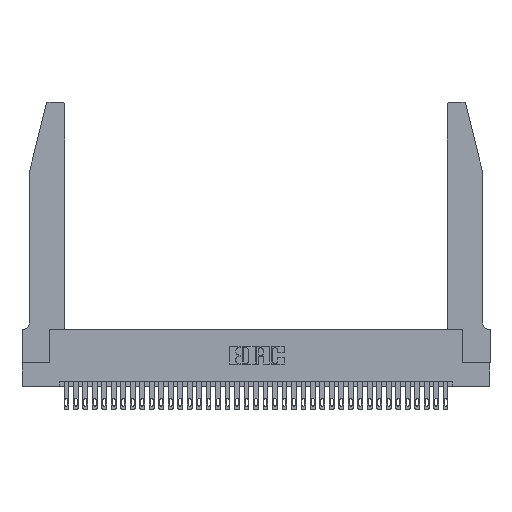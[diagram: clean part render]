
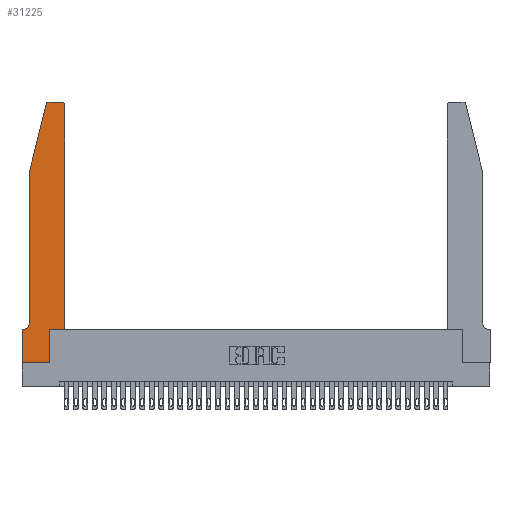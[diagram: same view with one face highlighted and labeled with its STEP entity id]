
A CAD part, top view. The second image highlights one B-rep face of the part: STEP entity #31225.
In plain terms, the highlighted planar face has unit normal (0, 0, 1).
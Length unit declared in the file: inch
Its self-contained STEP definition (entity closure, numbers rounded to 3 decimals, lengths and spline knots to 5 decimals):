
#162 = LINE ( 'NONE', #22549, #29637 ) ;
#183 = DIRECTION ( 'NONE',  ( 0., -1., 0. ) ) ;
#596 = CARTESIAN_POINT ( 'NONE',  ( 0.4205, 2.72, 0.37 ) ) ;
#1191 = VERTEX_POINT ( 'NONE', #33438 ) ;
#1701 = EDGE_CURVE ( 'NONE', #1191, #5198, #1761, .T. ) ;
#1761 = LINE ( 'NONE', #12296, #34817 ) ;
#2145 = VECTOR ( 'NONE', #18268, 39.37008 ) ;
#2172 = CIRCLE ( 'NONE', #9292, 0.03 ) ;
#2718 = VECTOR ( 'NONE', #27324, 39.37008 ) ;
#3950 = CARTESIAN_POINT ( 'NONE',  ( 0.2865, 0., 0.37 ) ) ;
#4523 = LINE ( 'NONE', #21981, #15677 ) ;
#5197 = DIRECTION ( 'NONE',  ( -0.239, -0.971, 0. ) ) ;
#5198 = VERTEX_POINT ( 'NONE', #32969 ) ;
#5276 = ORIENTED_EDGE ( 'NONE', *, *, #17188, .T. ) ;
#6531 = DIRECTION ( 'NONE',  ( 1., 0., 0. ) ) ;
#6892 = EDGE_CURVE ( 'NONE', #14827, #27369, #30427, .T. ) ;
#7015 = CARTESIAN_POINT ( 'NONE',  ( 0.0055, 0.42, 0.37 ) ) ;
#7888 = DIRECTION ( 'NONE',  ( 0., -1., 0. ) ) ;
#8024 = LINE ( 'NONE', #29529, #2145 ) ;
#8298 = CARTESIAN_POINT ( 'NONE',  ( 0.0755, 2., 0.37 ) ) ;
#9032 = ORIENTED_EDGE ( 'NONE', *, *, #20351, .T. ) ;
#9292 = AXIS2_PLACEMENT_3D ( 'NONE', #596, #12249, #28972 ) ;
#9358 = AXIS2_PLACEMENT_3D ( 'NONE', #20378, #23375, #6531 ) ;
#10999 = CIRCLE ( 'NONE', #25867, 0.07 ) ;
#11625 = LINE ( 'NONE', #24197, #2718 ) ;
#12249 = DIRECTION ( 'NONE',  ( 0., 0., 1. ) ) ;
#12296 = CARTESIAN_POINT ( 'NONE',  ( 0.2605, 2.75, 0.37 ) ) ;
#12471 = VERTEX_POINT ( 'NONE', #14321 ) ;
#13964 = CARTESIAN_POINT ( 'NONE',  ( 0.4505, 0.35, 0.37 ) ) ;
#14091 = DIRECTION ( 'NONE',  ( 1., 0., 0. ) ) ;
#14196 = ORIENTED_EDGE ( 'NONE', *, *, #32688, .T. ) ;
#14321 = CARTESIAN_POINT ( 'NONE',  ( 0., 0.35, 0.37 ) ) ;
#14362 = ORIENTED_EDGE ( 'NONE', *, *, #1701, .T. ) ;
#14827 = VERTEX_POINT ( 'NONE', #35647 ) ;
#15459 = CARTESIAN_POINT ( 'NONE',  ( 0.4505, 2.72, 0.37 ) ) ;
#15597 = VECTOR ( 'NONE', #14091, 39.37008 ) ;
#15677 = VECTOR ( 'NONE', #5197, 39.37008 ) ;
#15746 = DIRECTION ( 'NONE',  ( 0., 0., -1. ) ) ;
#15808 = VERTEX_POINT ( 'NONE', #15459 ) ;
#15870 = CARTESIAN_POINT ( 'NONE',  ( 0.25487, 2.72718, 0.37 ) ) ;
#17188 = EDGE_CURVE ( 'NONE', #22507, #15808, #11625, .T. ) ;
#17526 = EDGE_CURVE ( 'NONE', #23054, #22507, #30840, .T. ) ;
#18078 = AXIS2_PLACEMENT_3D ( 'NONE', #24322, #18310, #26941 ) ;
#18230 = VERTEX_POINT ( 'NONE', #27819 ) ;
#18268 = DIRECTION ( 'NONE',  ( -1., 0., 0. ) ) ;
#18310 = DIRECTION ( 'NONE',  ( 0., 0., 1. ) ) ;
#19824 = CARTESIAN_POINT ( 'NONE',  ( 0.0755, 2., 0.37 ) ) ;
#20351 = EDGE_CURVE ( 'NONE', #27369, #23054, #162, .T. ) ;
#20378 = CARTESIAN_POINT ( 'NONE',  ( 0.284, 2.72, 0.37 ) ) ;
#20587 = VERTEX_POINT ( 'NONE', #21298 ) ;
#20626 = EDGE_CURVE ( 'NONE', #12471, #14827, #30163, .T. ) ;
#21061 = DIRECTION ( 'NONE',  ( -1., 0., 0. ) ) ;
#21205 = DIRECTION ( 'NONE',  ( 1., 0., 0. ) ) ;
#21298 = CARTESIAN_POINT ( 'NONE',  ( 0.0755, 0.42, 0.37 ) ) ;
#21981 = CARTESIAN_POINT ( 'NONE',  ( 0.0755, 2., 0.37 ) ) ;
#22446 = CARTESIAN_POINT ( 'NONE',  ( 0.4505, 0.35, 0.37 ) ) ;
#22507 = VERTEX_POINT ( 'NONE', #22446 ) ;
#22549 = CARTESIAN_POINT ( 'NONE',  ( 0.2865, 0.35, 0.37 ) ) ;
#22848 = ORIENTED_EDGE ( 'NONE', *, *, #34748, .T. ) ;
#23054 = VERTEX_POINT ( 'NONE', #26611 ) ;
#23058 = EDGE_CURVE ( 'NONE', #15808, #1191, #2172, .T. ) ;
#23165 = CIRCLE ( 'NONE', #9358, 0.03 ) ;
#23209 = VECTOR ( 'NONE', #21205, 39.37008 ) ;
#23375 = DIRECTION ( 'NONE',  ( 0., 0., 1. ) ) ;
#23761 = DIRECTION ( 'NONE',  ( -1., 0., 0. ) ) ;
#23992 = ORIENTED_EDGE ( 'NONE', *, *, #35202, .T. ) ;
#24197 = CARTESIAN_POINT ( 'NONE',  ( 0.4505, 0.35, 0.37 ) ) ;
#24256 = EDGE_CURVE ( 'NONE', #18230, #12471, #8024, .T. ) ;
#24322 = CARTESIAN_POINT ( 'NONE',  ( 0., 0.35, 0.37 ) ) ;
#24709 = ORIENTED_EDGE ( 'NONE', *, *, #6892, .T. ) ;
#24815 = CARTESIAN_POINT ( 'NONE',  ( 0., 0., 0.37 ) ) ;
#25210 = EDGE_LOOP ( 'NONE', ( #14362, #23992, #32655, #22848, #14196, #31084, #29893, #24709, #9032, #28536, #5276, #34624 ) ) ;
#25377 = FACE_OUTER_BOUND ( 'NONE', #25210, .T. ) ;
#25867 = AXIS2_PLACEMENT_3D ( 'NONE', #7015, #15746, #21061 ) ;
#26611 = CARTESIAN_POINT ( 'NONE',  ( 0.2865, 0.35, 0.37 ) ) ;
#26941 = DIRECTION ( 'NONE',  ( 1., 0., 0. ) ) ;
#27324 = DIRECTION ( 'NONE',  ( 0., 1., 0. ) ) ;
#27369 = VERTEX_POINT ( 'NONE', #3950 ) ;
#27718 = LINE ( 'NONE', #8298, #36687 ) ;
#27819 = CARTESIAN_POINT ( 'NONE',  ( 0.0055, 0.35, 0.37 ) ) ;
#28536 = ORIENTED_EDGE ( 'NONE', *, *, #17526, .T. ) ;
#28728 = EDGE_CURVE ( 'NONE', #35998, #35074, #4523, .T. ) ;
#28972 = DIRECTION ( 'NONE',  ( 1., 0., 0. ) ) ;
#29529 = CARTESIAN_POINT ( 'NONE',  ( 0.0755, 0.35, 0.37 ) ) ;
#29637 = VECTOR ( 'NONE', #34060, 39.37008 ) ;
#29893 = ORIENTED_EDGE ( 'NONE', *, *, #20626, .T. ) ;
#29977 = CARTESIAN_POINT ( 'NONE',  ( 0., 0., 0.37 ) ) ;
#30163 = LINE ( 'NONE', #24815, #36206 ) ;
#30427 = LINE ( 'NONE', #29977, #23209 ) ;
#30840 = LINE ( 'NONE', #13964, #15597 ) ;
#31084 = ORIENTED_EDGE ( 'NONE', *, *, #24256, .T. ) ;
#31225 = ADVANCED_FACE ( 'NONE', ( #25377 ), #35408, .T. ) ;
#32655 = ORIENTED_EDGE ( 'NONE', *, *, #28728, .T. ) ;
#32688 = EDGE_CURVE ( 'NONE', #20587, #18230, #10999, .T. ) ;
#32969 = CARTESIAN_POINT ( 'NONE',  ( 0.284, 2.75, 0.37 ) ) ;
#33438 = CARTESIAN_POINT ( 'NONE',  ( 0.4205, 2.75, 0.37 ) ) ;
#34060 = DIRECTION ( 'NONE',  ( 0., 1., 0. ) ) ;
#34624 = ORIENTED_EDGE ( 'NONE', *, *, #23058, .T. ) ;
#34748 = EDGE_CURVE ( 'NONE', #35074, #20587, #27718, .T. ) ;
#34817 = VECTOR ( 'NONE', #23761, 39.37008 ) ;
#35074 = VERTEX_POINT ( 'NONE', #19824 ) ;
#35202 = EDGE_CURVE ( 'NONE', #5198, #35998, #23165, .T. ) ;
#35408 = PLANE ( 'NONE',  #18078 ) ;
#35647 = CARTESIAN_POINT ( 'NONE',  ( 0., 0., 0.37 ) ) ;
#35998 = VERTEX_POINT ( 'NONE', #15870 ) ;
#36206 = VECTOR ( 'NONE', #7888, 39.37008 ) ;
#36687 = VECTOR ( 'NONE', #183, 39.37008 ) ;
